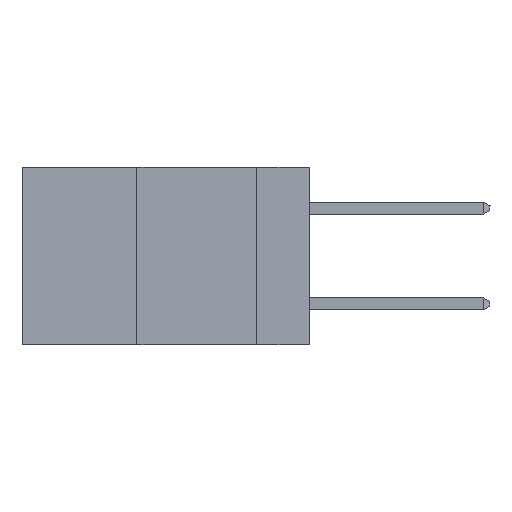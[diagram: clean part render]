
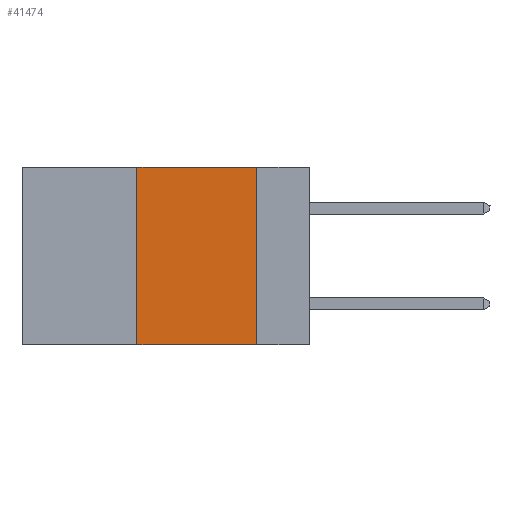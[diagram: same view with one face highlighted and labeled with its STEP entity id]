
A CAD part, left-side view. The second image highlights one B-rep face of the part: STEP entity #41474.
In plain terms, the highlighted planar face has unit normal (-1, 0, 0).
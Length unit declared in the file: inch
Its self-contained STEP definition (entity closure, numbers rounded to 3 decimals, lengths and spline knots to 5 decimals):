
#667 = AXIS2_PLACEMENT_3D ( 'NONE', #17764, #30770, #10729 ) ;
#712 = CARTESIAN_POINT ( 'NONE',  ( 0., 0.6, -0.37 ) ) ;
#886 = CARTESIAN_POINT ( 'NONE',  ( 0., 0.11, -0.37 ) ) ;
#1063 = CARTESIAN_POINT ( 'NONE',  ( 0., 0.11, 0. ) ) ;
#3876 = VERTEX_POINT ( 'NONE', #6128 ) ;
#5019 = CARTESIAN_POINT ( 'NONE',  ( 0., 0.36, 0. ) ) ;
#6128 = CARTESIAN_POINT ( 'NONE',  ( 0., 0.11, 0. ) ) ;
#7034 = VECTOR ( 'NONE', #11914, 39.37008 ) ;
#7908 = EDGE_CURVE ( 'NONE', #19394, #10438, #25403, .T. ) ;
#9488 = ORIENTED_EDGE ( 'NONE', *, *, #26584, .F. ) ;
#10438 = VERTEX_POINT ( 'NONE', #28051 ) ;
#10729 = DIRECTION ( 'NONE',  ( 0., 0., -1. ) ) ;
#11027 = DIRECTION ( 'NONE',  ( 0., -1., 0. ) ) ;
#11223 = DIRECTION ( 'NONE',  ( 0., 0., -1. ) ) ;
#11499 = ORIENTED_EDGE ( 'NONE', *, *, #18310, .T. ) ;
#11914 = DIRECTION ( 'NONE',  ( 0., 0., 1. ) ) ;
#12111 = CARTESIAN_POINT ( 'NONE',  ( 0., 0.6, 0. ) ) ;
#15517 = DIRECTION ( 'NONE',  ( 0., -1., 0. ) ) ;
#17764 = CARTESIAN_POINT ( 'NONE',  ( 0., 0.6, 0. ) ) ;
#18087 = LINE ( 'NONE', #1063, #31173 ) ;
#18310 = EDGE_CURVE ( 'NONE', #19394, #36457, #37417, .T. ) ;
#19394 = VERTEX_POINT ( 'NONE', #39714 ) ;
#23000 = EDGE_CURVE ( 'NONE', #3876, #36457, #18087, .T. ) ;
#24210 = EDGE_LOOP ( 'NONE', ( #32666, #9488, #32489, #11499 ) ) ;
#25403 = LINE ( 'NONE', #5019, #7034 ) ;
#26584 = EDGE_CURVE ( 'NONE', #10438, #3876, #38899, .T. ) ;
#27817 = VECTOR ( 'NONE', #15517, 39.37008 ) ;
#28051 = CARTESIAN_POINT ( 'NONE',  ( 0., 0.36, 0. ) ) ;
#30770 = DIRECTION ( 'NONE',  ( 1., 0., 0. ) ) ;
#31173 = VECTOR ( 'NONE', #11223, 39.37008 ) ;
#32489 = ORIENTED_EDGE ( 'NONE', *, *, #7908, .F. ) ;
#32666 = ORIENTED_EDGE ( 'NONE', *, *, #23000, .F. ) ;
#34294 = VECTOR ( 'NONE', #11027, 39.37008 ) ;
#36457 = VERTEX_POINT ( 'NONE', #886 ) ;
#37417 = LINE ( 'NONE', #712, #34294 ) ;
#37788 = PLANE ( 'NONE',  #667 ) ;
#38899 = LINE ( 'NONE', #12111, #27817 ) ;
#39178 = FACE_OUTER_BOUND ( 'NONE', #24210, .T. ) ;
#39714 = CARTESIAN_POINT ( 'NONE',  ( 0., 0.36, -0.37 ) ) ;
#41474 = ADVANCED_FACE ( 'NONE', ( #39178 ), #37788, .F. ) ;
